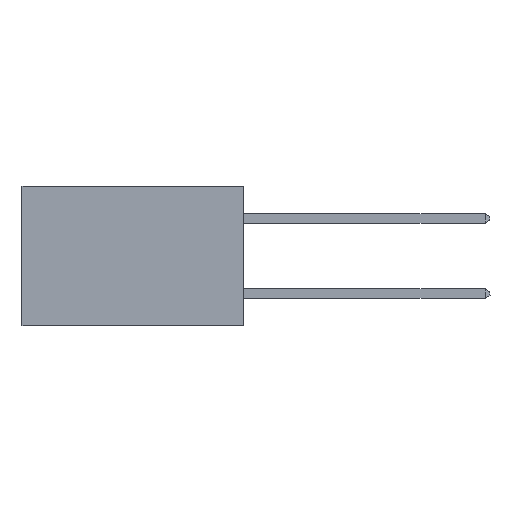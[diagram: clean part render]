
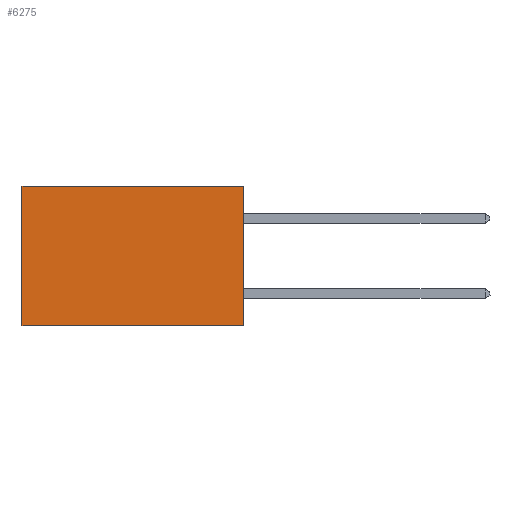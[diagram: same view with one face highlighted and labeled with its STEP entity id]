
A CAD part, left-side view. The second image highlights one B-rep face of the part: STEP entity #6275.
In plain terms, the highlighted planar face has unit normal (-1, 0, 0).
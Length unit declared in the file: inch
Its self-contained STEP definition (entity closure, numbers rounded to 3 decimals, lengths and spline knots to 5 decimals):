
#620 = FACE_OUTER_BOUND ( 'NONE', #2877, .T. ) ;
#897 = VERTEX_POINT ( 'NONE', #4661 ) ;
#1553 = DIRECTION ( 'NONE',  ( 0., 0., -1. ) ) ;
#2217 = VECTOR ( 'NONE', #9472, 39.37008 ) ;
#2685 = CARTESIAN_POINT ( 'NONE',  ( 0.277, 0., -0.37 ) ) ;
#2877 = EDGE_LOOP ( 'NONE', ( #6037, #4889, #5464, #3633 ) ) ;
#2910 = DIRECTION ( 'NONE',  ( 0., 0., -1. ) ) ;
#2912 = DIRECTION ( 'NONE',  ( 1., 0., 0. ) ) ;
#2925 = PLANE ( 'NONE',  #7762 ) ;
#2977 = CARTESIAN_POINT ( 'NONE',  ( 0.277, 0., -0.37 ) ) ;
#3128 = EDGE_CURVE ( 'NONE', #897, #5984, #7277, .T. ) ;
#3153 = EDGE_CURVE ( 'NONE', #897, #3470, #11481, .T. ) ;
#3230 = LINE ( 'NONE', #10622, #3539 ) ;
#3470 = VERTEX_POINT ( 'NONE', #4243 ) ;
#3539 = VECTOR ( 'NONE', #1553, 39.37008 ) ;
#3633 = ORIENTED_EDGE ( 'NONE', *, *, #3153, .T. ) ;
#4243 = CARTESIAN_POINT ( 'NONE',  ( 0.277, 0.59, 0. ) ) ;
#4661 = CARTESIAN_POINT ( 'NONE',  ( 0.277, 0., 0. ) ) ;
#4665 = CARTESIAN_POINT ( 'NONE',  ( 0.277, 0., -0.37 ) ) ;
#4751 = VERTEX_POINT ( 'NONE', #11067 ) ;
#4889 = ORIENTED_EDGE ( 'NONE', *, *, #10318, .F. ) ;
#5464 = ORIENTED_EDGE ( 'NONE', *, *, #3128, .F. ) ;
#5984 = VERTEX_POINT ( 'NONE', #4665 ) ;
#6037 = ORIENTED_EDGE ( 'NONE', *, *, #11516, .T. ) ;
#6275 = ADVANCED_FACE ( 'NONE', ( #620 ), #2925, .F. ) ;
#6993 = VECTOR ( 'NONE', #7990, 39.37008 ) ;
#7277 = LINE ( 'NONE', #8317, #2217 ) ;
#7762 = AXIS2_PLACEMENT_3D ( 'NONE', #2977, #2912, #2910 ) ;
#7990 = DIRECTION ( 'NONE',  ( 0., 1., 0. ) ) ;
#8006 = CARTESIAN_POINT ( 'NONE',  ( 0.277, 0., 0. ) ) ;
#8317 = CARTESIAN_POINT ( 'NONE',  ( 0.277, 0., -0.37 ) ) ;
#8971 = LINE ( 'NONE', #2685, #10913 ) ;
#9472 = DIRECTION ( 'NONE',  ( 0., 0., -1. ) ) ;
#9966 = DIRECTION ( 'NONE',  ( 0., 1., 0. ) ) ;
#10318 = EDGE_CURVE ( 'NONE', #5984, #4751, #8971, .T. ) ;
#10622 = CARTESIAN_POINT ( 'NONE',  ( 0.277, 0.59, -0.37 ) ) ;
#10913 = VECTOR ( 'NONE', #9966, 39.37008 ) ;
#11067 = CARTESIAN_POINT ( 'NONE',  ( 0.277, 0.59, -0.37 ) ) ;
#11481 = LINE ( 'NONE', #8006, #6993 ) ;
#11516 = EDGE_CURVE ( 'NONE', #3470, #4751, #3230, .T. ) ;
